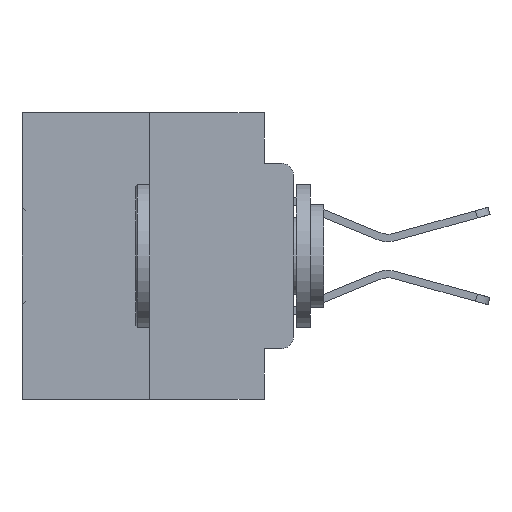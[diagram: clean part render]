
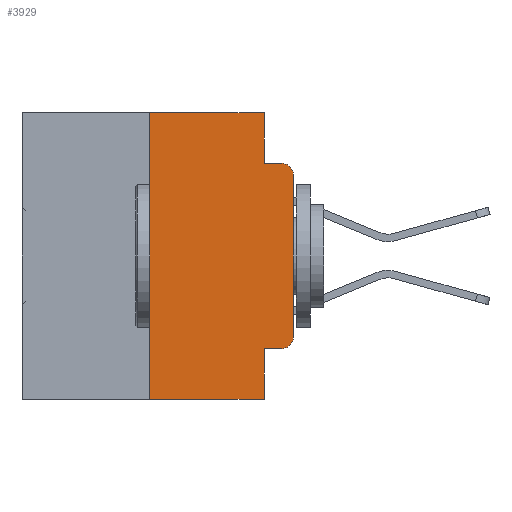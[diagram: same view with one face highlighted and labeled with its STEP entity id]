
A CAD part, left-side view. The second image highlights one B-rep face of the part: STEP entity #3929.
In plain terms, the highlighted planar face has unit normal (-1, 0, 0).
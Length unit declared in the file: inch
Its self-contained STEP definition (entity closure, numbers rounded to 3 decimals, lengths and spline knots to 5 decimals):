
#1709 = LINE ( 'NONE', #11575, #28510 ) ;
#2299 = DIRECTION ( 'NONE',  ( 0., 0., 1. ) ) ;
#2477 = EDGE_CURVE ( 'NONE', #15529, #30112, #5296, .T. ) ;
#2653 = CARTESIAN_POINT ( 'NONE',  ( 0., 0.25, 0. ) ) ;
#2713 = VERTEX_POINT ( 'NONE', #18750 ) ;
#3328 = LINE ( 'NONE', #17271, #16391 ) ;
#3732 = VERTEX_POINT ( 'NONE', #15895 ) ;
#3902 = DIRECTION ( 'NONE',  ( 0., 0., 1. ) ) ;
#3929 = ADVANCED_FACE ( 'NONE', ( #25356 ), #16012, .F. ) ;
#4225 = DIRECTION ( 'NONE',  ( 0., -1., 0. ) ) ;
#4874 = CARTESIAN_POINT ( 'NONE',  ( 0., 0.02, -0.0885 ) ) ;
#5296 = CIRCLE ( 'NONE', #32200, 0.02 ) ;
#5672 = EDGE_LOOP ( 'NONE', ( #16873, #6229, #28550, #23349, #26560, #15217, #23775, #26967, #28582, #12744 ) ) ;
#6229 = ORIENTED_EDGE ( 'NONE', *, *, #23517, .T. ) ;
#6284 = CARTESIAN_POINT ( 'NONE',  ( 0., 0., -0.1085 ) ) ;
#6302 = VERTEX_POINT ( 'NONE', #6284 ) ;
#6817 = CARTESIAN_POINT ( 'NONE',  ( 0., 0.473, -0.5 ) ) ;
#7000 = CARTESIAN_POINT ( 'NONE',  ( 0., 0.051, -0.5 ) ) ;
#7705 = VECTOR ( 'NONE', #4225, 39.37008 ) ;
#8508 = VERTEX_POINT ( 'NONE', #16739 ) ;
#9139 = VERTEX_POINT ( 'NONE', #29766 ) ;
#9246 = EDGE_CURVE ( 'NONE', #8508, #2713, #3328, .T. ) ;
#9670 = CARTESIAN_POINT ( 'NONE',  ( 0., 0.051, 0. ) ) ;
#9839 = EDGE_CURVE ( 'NONE', #3732, #15529, #27632, .T. ) ;
#10444 = CARTESIAN_POINT ( 'NONE',  ( 0., 0.02, -0.1085 ) ) ;
#11311 = VECTOR ( 'NONE', #15126, 39.37008 ) ;
#11409 = LINE ( 'NONE', #30286, #31280 ) ;
#11575 = CARTESIAN_POINT ( 'NONE',  ( 0., 0., 0. ) ) ;
#12121 = DIRECTION ( 'NONE',  ( 0., -1., 0. ) ) ;
#12306 = DIRECTION ( 'NONE',  ( 0., 0., -1. ) ) ;
#12666 = CARTESIAN_POINT ( 'NONE',  ( 0., 0.02, -0.3915 ) ) ;
#12744 = ORIENTED_EDGE ( 'NONE', *, *, #2477, .T. ) ;
#12994 = VECTOR ( 'NONE', #24661, 39.37008 ) ;
#13066 = DIRECTION ( 'NONE',  ( 0., 0., -1. ) ) ;
#13095 = DIRECTION ( 'NONE',  ( 1., 0., 0. ) ) ;
#13404 = DIRECTION ( 'NONE',  ( 0., 0., -1. ) ) ;
#15126 = DIRECTION ( 'NONE',  ( 0., -1., 0. ) ) ;
#15217 = ORIENTED_EDGE ( 'NONE', *, *, #28612, .F. ) ;
#15241 = EDGE_CURVE ( 'NONE', #30112, #6302, #1709, .T. ) ;
#15529 = VERTEX_POINT ( 'NONE', #18048 ) ;
#15621 = CARTESIAN_POINT ( 'NONE',  ( 0., 0.473, 0. ) ) ;
#15760 = VECTOR ( 'NONE', #12306, 39.37008 ) ;
#15895 = CARTESIAN_POINT ( 'NONE',  ( 0., 0.051, -0.4115 ) ) ;
#16012 = PLANE ( 'NONE',  #24584 ) ;
#16212 = DIRECTION ( 'NONE',  ( -1., 0., 0. ) ) ;
#16251 = DIRECTION ( 'NONE',  ( 0., 0., -1. ) ) ;
#16391 = VECTOR ( 'NONE', #19892, 39.37008 ) ;
#16739 = CARTESIAN_POINT ( 'NONE',  ( 0., 0.051, 0. ) ) ;
#16850 = VERTEX_POINT ( 'NONE', #4874 ) ;
#16873 = ORIENTED_EDGE ( 'NONE', *, *, #15241, .T. ) ;
#17271 = CARTESIAN_POINT ( 'NONE',  ( 0., 0.051, 0. ) ) ;
#17962 = CARTESIAN_POINT ( 'NONE',  ( 0., 0.25, 0. ) ) ;
#18048 = CARTESIAN_POINT ( 'NONE',  ( 0., 0.02, -0.4115 ) ) ;
#18377 = LINE ( 'NONE', #25445, #11311 ) ;
#18603 = LINE ( 'NONE', #17962, #22207 ) ;
#18750 = CARTESIAN_POINT ( 'NONE',  ( 0., 0.051, -0.0885 ) ) ;
#19049 = AXIS2_PLACEMENT_3D ( 'NONE', #10444, #28630, #13066 ) ;
#19892 = DIRECTION ( 'NONE',  ( 0., 0., -1. ) ) ;
#20426 = EDGE_CURVE ( 'NONE', #3732, #24556, #22679, .T. ) ;
#22104 = CARTESIAN_POINT ( 'NONE',  ( 0., 0.051, -0.4115 ) ) ;
#22207 = VECTOR ( 'NONE', #2299, 39.37008 ) ;
#22679 = LINE ( 'NONE', #9670, #15760 ) ;
#23349 = ORIENTED_EDGE ( 'NONE', *, *, #9246, .F. ) ;
#23415 = CIRCLE ( 'NONE', #19049, 0.02 ) ;
#23517 = EDGE_CURVE ( 'NONE', #6302, #16850, #23415, .T. ) ;
#23775 = ORIENTED_EDGE ( 'NONE', *, *, #32152, .T. ) ;
#24556 = VERTEX_POINT ( 'NONE', #7000 ) ;
#24584 = AXIS2_PLACEMENT_3D ( 'NONE', #15621, #13095, #16251 ) ;
#24661 = DIRECTION ( 'NONE',  ( 0., -1., 0. ) ) ;
#25356 = FACE_OUTER_BOUND ( 'NONE', #5672, .T. ) ;
#25445 = CARTESIAN_POINT ( 'NONE',  ( 0., 0.051, -0.0885 ) ) ;
#26560 = ORIENTED_EDGE ( 'NONE', *, *, #31010, .F. ) ;
#26967 = ORIENTED_EDGE ( 'NONE', *, *, #20426, .F. ) ;
#27632 = LINE ( 'NONE', #22104, #12994 ) ;
#28386 = LINE ( 'NONE', #6817, #7705 ) ;
#28510 = VECTOR ( 'NONE', #3902, 39.37008 ) ;
#28550 = ORIENTED_EDGE ( 'NONE', *, *, #32272, .F. ) ;
#28582 = ORIENTED_EDGE ( 'NONE', *, *, #9839, .T. ) ;
#28612 = EDGE_CURVE ( 'NONE', #9139, #28707, #18603, .T. ) ;
#28630 = DIRECTION ( 'NONE',  ( -1., 0., 0. ) ) ;
#28707 = VERTEX_POINT ( 'NONE', #2653 ) ;
#29766 = CARTESIAN_POINT ( 'NONE',  ( 0., 0.25, -0.5 ) ) ;
#30112 = VERTEX_POINT ( 'NONE', #32095 ) ;
#30286 = CARTESIAN_POINT ( 'NONE',  ( 0., 0.473, 0. ) ) ;
#31010 = EDGE_CURVE ( 'NONE', #28707, #8508, #11409, .T. ) ;
#31280 = VECTOR ( 'NONE', #12121, 39.37008 ) ;
#32095 = CARTESIAN_POINT ( 'NONE',  ( 0., 0., -0.3915 ) ) ;
#32152 = EDGE_CURVE ( 'NONE', #9139, #24556, #28386, .T. ) ;
#32200 = AXIS2_PLACEMENT_3D ( 'NONE', #12666, #16212, #13404 ) ;
#32272 = EDGE_CURVE ( 'NONE', #2713, #16850, #18377, .T. ) ;
